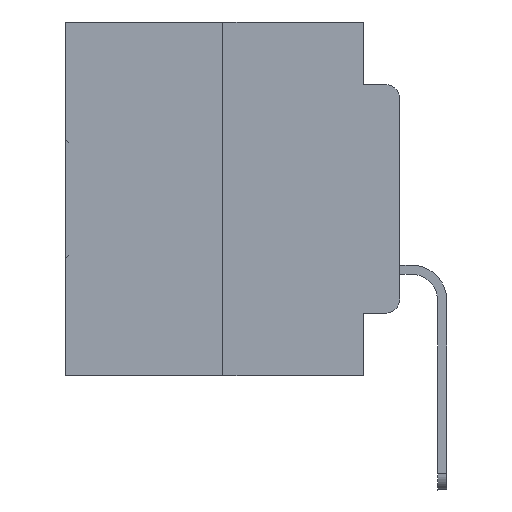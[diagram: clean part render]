
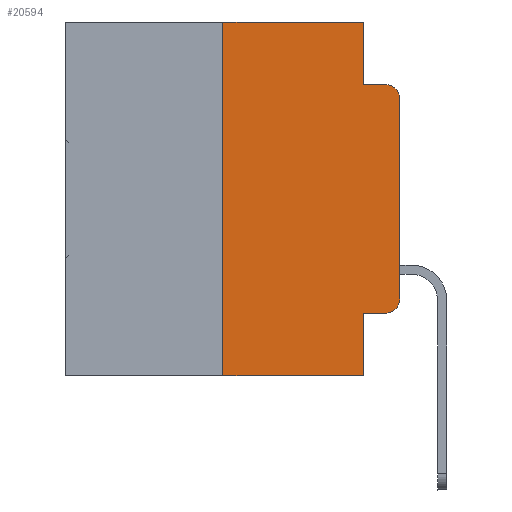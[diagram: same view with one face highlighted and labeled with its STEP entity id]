
A CAD part, left-side view. The second image highlights one B-rep face of the part: STEP entity #20594.
In plain terms, the highlighted planar face has unit normal (-1, 0, 0).
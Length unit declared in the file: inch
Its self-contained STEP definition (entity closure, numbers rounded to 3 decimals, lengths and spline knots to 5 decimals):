
#132 = DIRECTION ( 'NONE',  ( 0., 0., -1. ) ) ;
#299 = CIRCLE ( 'NONE', #18043, 0.02 ) ;
#391 = VERTEX_POINT ( 'NONE', #6401 ) ;
#432 = EDGE_CURVE ( 'NONE', #21816, #4360, #11469, .T. ) ;
#482 = LINE ( 'NONE', #12234, #26221 ) ;
#1042 = EDGE_CURVE ( 'NONE', #5203, #2519, #5145, .T. ) ;
#1046 = CARTESIAN_POINT ( 'NONE',  ( 0., 0.25, 0. ) ) ;
#2519 = VERTEX_POINT ( 'NONE', #21989 ) ;
#2835 = CARTESIAN_POINT ( 'NONE',  ( 0., 0., 0. ) ) ;
#3291 = CARTESIAN_POINT ( 'NONE',  ( 0., 0.02, -0.4115 ) ) ;
#3517 = AXIS2_PLACEMENT_3D ( 'NONE', #16065, #30526, #8788 ) ;
#3587 = CARTESIAN_POINT ( 'NONE',  ( 0., 0.02, -0.0885 ) ) ;
#4360 = VERTEX_POINT ( 'NONE', #8771 ) ;
#4490 = VECTOR ( 'NONE', #8221, 39.37008 ) ;
#4531 = ORIENTED_EDGE ( 'NONE', *, *, #12358, .F. ) ;
#4944 = VERTEX_POINT ( 'NONE', #28560 ) ;
#5145 = CIRCLE ( 'NONE', #27941, 0.02 ) ;
#5203 = VERTEX_POINT ( 'NONE', #3291 ) ;
#5767 = EDGE_CURVE ( 'NONE', #391, #14429, #22044, .T. ) ;
#6401 = CARTESIAN_POINT ( 'NONE',  ( 0., 0.051, -0.0885 ) ) ;
#6619 = LINE ( 'NONE', #16745, #10484 ) ;
#7262 = EDGE_CURVE ( 'NONE', #21816, #5203, #20015, .T. ) ;
#7780 = CARTESIAN_POINT ( 'NONE',  ( 0., 0.02, -0.3915 ) ) ;
#7828 = EDGE_CURVE ( 'NONE', #28513, #391, #11831, .T. ) ;
#8162 = ORIENTED_EDGE ( 'NONE', *, *, #27505, .T. ) ;
#8221 = DIRECTION ( 'NONE',  ( 0., 0., 1. ) ) ;
#8358 = VECTOR ( 'NONE', #22554, 39.37008 ) ;
#8771 = CARTESIAN_POINT ( 'NONE',  ( 0., 0.051, -0.5 ) ) ;
#8788 = DIRECTION ( 'NONE',  ( 0., 0., -1. ) ) ;
#8971 = ORIENTED_EDGE ( 'NONE', *, *, #5767, .F. ) ;
#10002 = DIRECTION ( 'NONE',  ( 0., 0., -1. ) ) ;
#10172 = EDGE_CURVE ( 'NONE', #10985, #4360, #6619, .T. ) ;
#10449 = DIRECTION ( 'NONE',  ( 0., -1., 0. ) ) ;
#10459 = LINE ( 'NONE', #2835, #16661 ) ;
#10484 = VECTOR ( 'NONE', #16270, 39.37008 ) ;
#10559 = VECTOR ( 'NONE', #10449, 39.37008 ) ;
#10985 = VERTEX_POINT ( 'NONE', #16627 ) ;
#11026 = CARTESIAN_POINT ( 'NONE',  ( 0., 0., -0.1085 ) ) ;
#11469 = LINE ( 'NONE', #18132, #17716 ) ;
#11831 = LINE ( 'NONE', #23580, #26122 ) ;
#12234 = CARTESIAN_POINT ( 'NONE',  ( 0., 0.473, 0. ) ) ;
#12338 = ORIENTED_EDGE ( 'NONE', *, *, #16900, .T. ) ;
#12358 = EDGE_CURVE ( 'NONE', #10985, #4944, #17251, .T. ) ;
#14135 = ORIENTED_EDGE ( 'NONE', *, *, #1042, .T. ) ;
#14418 = ORIENTED_EDGE ( 'NONE', *, *, #7828, .F. ) ;
#14429 = VERTEX_POINT ( 'NONE', #3587 ) ;
#16065 = CARTESIAN_POINT ( 'NONE',  ( 0., 0.473, 0. ) ) ;
#16270 = DIRECTION ( 'NONE',  ( 0., -1., 0. ) ) ;
#16627 = CARTESIAN_POINT ( 'NONE',  ( 0., 0.25, -0.5 ) ) ;
#16661 = VECTOR ( 'NONE', #20440, 39.37008 ) ;
#16681 = CARTESIAN_POINT ( 'NONE',  ( 0., 0.051, -0.4115 ) ) ;
#16745 = CARTESIAN_POINT ( 'NONE',  ( 0., 0.473, -0.5 ) ) ;
#16900 = EDGE_CURVE ( 'NONE', #22945, #14429, #299, .T. ) ;
#17251 = LINE ( 'NONE', #1046, #4490 ) ;
#17716 = VECTOR ( 'NONE', #21149, 39.37008 ) ;
#17725 = EDGE_CURVE ( 'NONE', #4944, #28513, #482, .T. ) ;
#18043 = AXIS2_PLACEMENT_3D ( 'NONE', #19838, #29527, #10002 ) ;
#18132 = CARTESIAN_POINT ( 'NONE',  ( 0., 0.051, 0. ) ) ;
#18788 = ORIENTED_EDGE ( 'NONE', *, *, #7262, .T. ) ;
#19838 = CARTESIAN_POINT ( 'NONE',  ( 0., 0.02, -0.1085 ) ) ;
#20015 = LINE ( 'NONE', #24953, #8358 ) ;
#20440 = DIRECTION ( 'NONE',  ( 0., 0., 1. ) ) ;
#20594 = ADVANCED_FACE ( 'NONE', ( #20841 ), #25924, .F. ) ;
#20841 = FACE_OUTER_BOUND ( 'NONE', #30476, .T. ) ;
#21149 = DIRECTION ( 'NONE',  ( 0., 0., -1. ) ) ;
#21816 = VERTEX_POINT ( 'NONE', #16681 ) ;
#21989 = CARTESIAN_POINT ( 'NONE',  ( 0., 0., -0.3915 ) ) ;
#22044 = LINE ( 'NONE', #29665, #10559 ) ;
#22244 = DIRECTION ( 'NONE',  ( 0., -1., 0. ) ) ;
#22554 = DIRECTION ( 'NONE',  ( 0., -1., 0. ) ) ;
#22945 = VERTEX_POINT ( 'NONE', #11026 ) ;
#23557 = ORIENTED_EDGE ( 'NONE', *, *, #432, .F. ) ;
#23580 = CARTESIAN_POINT ( 'NONE',  ( 0., 0.051, 0. ) ) ;
#24953 = CARTESIAN_POINT ( 'NONE',  ( 0., 0.051, -0.4115 ) ) ;
#25643 = ORIENTED_EDGE ( 'NONE', *, *, #10172, .T. ) ;
#25924 = PLANE ( 'NONE',  #3517 ) ;
#25975 = ORIENTED_EDGE ( 'NONE', *, *, #17725, .F. ) ;
#26122 = VECTOR ( 'NONE', #26432, 39.37008 ) ;
#26221 = VECTOR ( 'NONE', #22244, 39.37008 ) ;
#26432 = DIRECTION ( 'NONE',  ( 0., 0., -1. ) ) ;
#27505 = EDGE_CURVE ( 'NONE', #2519, #22945, #10459, .T. ) ;
#27941 = AXIS2_PLACEMENT_3D ( 'NONE', #7780, #29363, #132 ) ;
#28102 = CARTESIAN_POINT ( 'NONE',  ( 0., 0.051, 0. ) ) ;
#28513 = VERTEX_POINT ( 'NONE', #28102 ) ;
#28560 = CARTESIAN_POINT ( 'NONE',  ( 0., 0.25, 0. ) ) ;
#29363 = DIRECTION ( 'NONE',  ( -1., 0., 0. ) ) ;
#29527 = DIRECTION ( 'NONE',  ( -1., 0., 0. ) ) ;
#29665 = CARTESIAN_POINT ( 'NONE',  ( 0., 0.051, -0.0885 ) ) ;
#30476 = EDGE_LOOP ( 'NONE', ( #8162, #12338, #8971, #14418, #25975, #4531, #25643, #23557, #18788, #14135 ) ) ;
#30526 = DIRECTION ( 'NONE',  ( 1., 0., 0. ) ) ;
